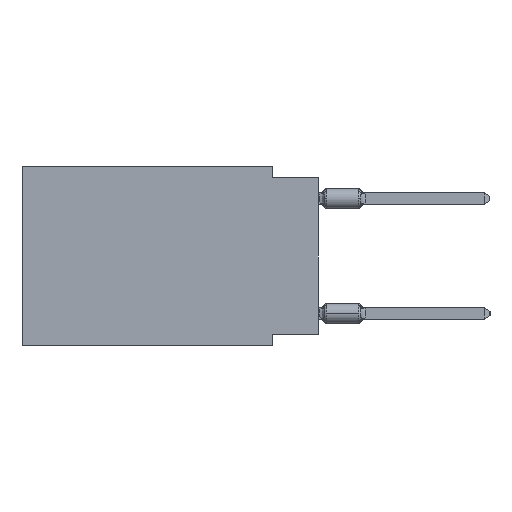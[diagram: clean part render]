
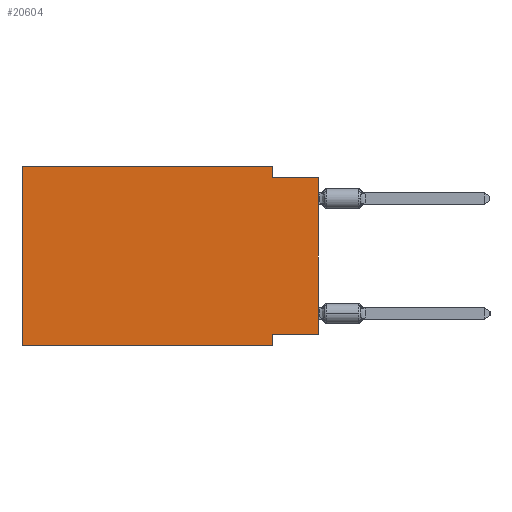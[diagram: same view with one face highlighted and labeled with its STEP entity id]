
A CAD part, left-side view. The second image highlights one B-rep face of the part: STEP entity #20604.
In plain terms, the highlighted planar face has unit normal (-1, 0, 0).
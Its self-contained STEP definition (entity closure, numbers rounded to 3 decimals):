
#49 = CARTESIAN_POINT ( 'NONE',  ( 0., 2.54, -9.906 ) ) ;
#360 = PLANE ( 'NONE',  #16449 ) ;
#1447 = EDGE_CURVE ( 'NONE', #50260, #48572, #22486, .T. ) ;
#4201 = LINE ( 'NONE', #15558, #40764 ) ;
#4315 = ORIENTED_EDGE ( 'NONE', *, *, #29855, .T. ) ;
#4807 = CARTESIAN_POINT ( 'NONE',  ( 0., 2.54, 0. ) ) ;
#5285 = VERTEX_POINT ( 'NONE', #42399 ) ;
#5335 = DIRECTION ( 'NONE',  ( 0., 0., 1. ) ) ;
#5378 = CARTESIAN_POINT ( 'NONE',  ( 0., 2.54, 0. ) ) ;
#8037 = ORIENTED_EDGE ( 'NONE', *, *, #48336, .F. ) ;
#8467 = ORIENTED_EDGE ( 'NONE', *, *, #18324, .F. ) ;
#10207 = CARTESIAN_POINT ( 'NONE',  ( 0., 2.54, -0.635 ) ) ;
#10486 = ORIENTED_EDGE ( 'NONE', *, *, #17141, .F. ) ;
#13262 = CARTESIAN_POINT ( 'NONE',  ( 0., 16.383, 0. ) ) ;
#14079 = CARTESIAN_POINT ( 'NONE',  ( 0., 0., -9.271 ) ) ;
#15003 = CARTESIAN_POINT ( 'NONE',  ( 0., 16.383, -9.906 ) ) ;
#15558 = CARTESIAN_POINT ( 'NONE',  ( 0., 0., -0.635 ) ) ;
#16449 = AXIS2_PLACEMENT_3D ( 'NONE', #13262, #32278, #36771 ) ;
#17141 = EDGE_CURVE ( 'NONE', #41049, #5285, #4201, .T. ) ;
#17255 = LINE ( 'NONE', #5378, #40761 ) ;
#18324 = EDGE_CURVE ( 'NONE', #35552, #41049, #17255, .T. ) ;
#19253 = ORIENTED_EDGE ( 'NONE', *, *, #29490, .F. ) ;
#19641 = VERTEX_POINT ( 'NONE', #33263 ) ;
#20604 = ADVANCED_FACE ( 'NONE', ( #45210 ), #360, .F. ) ;
#21231 = LINE ( 'NONE', #37357, #26579 ) ;
#21985 = DIRECTION ( 'NONE',  ( 0., 0., -1. ) ) ;
#22486 = LINE ( 'NONE', #42316, #34321 ) ;
#22821 = ORIENTED_EDGE ( 'NONE', *, *, #1447, .F. ) ;
#23687 = LINE ( 'NONE', #15003, #36479 ) ;
#24766 = ORIENTED_EDGE ( 'NONE', *, *, #27652, .F. ) ;
#24933 = DIRECTION ( 'NONE',  ( 0., 0., -1. ) ) ;
#25651 = CARTESIAN_POINT ( 'NONE',  ( 0., 0., 0. ) ) ;
#25800 = CARTESIAN_POINT ( 'NONE',  ( 0., 16.383, 0. ) ) ;
#26150 = ORIENTED_EDGE ( 'NONE', *, *, #38513, .T. ) ;
#26579 = VECTOR ( 'NONE', #24933, 1000. ) ;
#27652 = EDGE_CURVE ( 'NONE', #36252, #19641, #38269, .T. ) ;
#27661 = LINE ( 'NONE', #36128, #51774 ) ;
#27808 = CARTESIAN_POINT ( 'NONE',  ( 0., 16.383, -9.906 ) ) ;
#29490 = EDGE_CURVE ( 'NONE', #19641, #49622, #21231, .T. ) ;
#29855 = EDGE_CURVE ( 'NONE', #36252, #5285, #32790, .T. ) ;
#32278 = DIRECTION ( 'NONE',  ( 1., 0., 0. ) ) ;
#32790 = LINE ( 'NONE', #25651, #35028 ) ;
#33263 = CARTESIAN_POINT ( 'NONE',  ( 0., 2.54, -9.271 ) ) ;
#33856 = DIRECTION ( 'NONE',  ( 0., 0., 1. ) ) ;
#34321 = VECTOR ( 'NONE', #33856, 1000. ) ;
#35028 = VECTOR ( 'NONE', #5335, 1000. ) ;
#35552 = VERTEX_POINT ( 'NONE', #4807 ) ;
#36128 = CARTESIAN_POINT ( 'NONE',  ( 0., 16.383, 0. ) ) ;
#36252 = VERTEX_POINT ( 'NONE', #14079 ) ;
#36479 = VECTOR ( 'NONE', #43258, 1000. ) ;
#36771 = DIRECTION ( 'NONE',  ( 0., 0., -1. ) ) ;
#37357 = CARTESIAN_POINT ( 'NONE',  ( 0., 2.54, -9.906 ) ) ;
#37487 = CARTESIAN_POINT ( 'NONE',  ( 0., 0., -9.271 ) ) ;
#38269 = LINE ( 'NONE', #37487, #50712 ) ;
#38513 = EDGE_CURVE ( 'NONE', #50260, #49622, #23687, .T. ) ;
#38522 = DIRECTION ( 'NONE',  ( 0., 1., 0. ) ) ;
#39830 = DIRECTION ( 'NONE',  ( 0., -1., 0. ) ) ;
#40761 = VECTOR ( 'NONE', #21985, 1000. ) ;
#40764 = VECTOR ( 'NONE', #48031, 1000. ) ;
#41049 = VERTEX_POINT ( 'NONE', #10207 ) ;
#42316 = CARTESIAN_POINT ( 'NONE',  ( 0., 16.383, 0. ) ) ;
#42399 = CARTESIAN_POINT ( 'NONE',  ( 0., 0., -0.635 ) ) ;
#43258 = DIRECTION ( 'NONE',  ( 0., -1., 0. ) ) ;
#45210 = FACE_OUTER_BOUND ( 'NONE', #51389, .T. ) ;
#48031 = DIRECTION ( 'NONE',  ( 0., -1., 0. ) ) ;
#48336 = EDGE_CURVE ( 'NONE', #48572, #35552, #27661, .T. ) ;
#48572 = VERTEX_POINT ( 'NONE', #25800 ) ;
#49622 = VERTEX_POINT ( 'NONE', #49 ) ;
#50260 = VERTEX_POINT ( 'NONE', #27808 ) ;
#50712 = VECTOR ( 'NONE', #38522, 1000. ) ;
#51389 = EDGE_LOOP ( 'NONE', ( #4315, #10486, #8467, #8037, #22821, #26150, #19253, #24766 ) ) ;
#51774 = VECTOR ( 'NONE', #39830, 1000. ) ;
